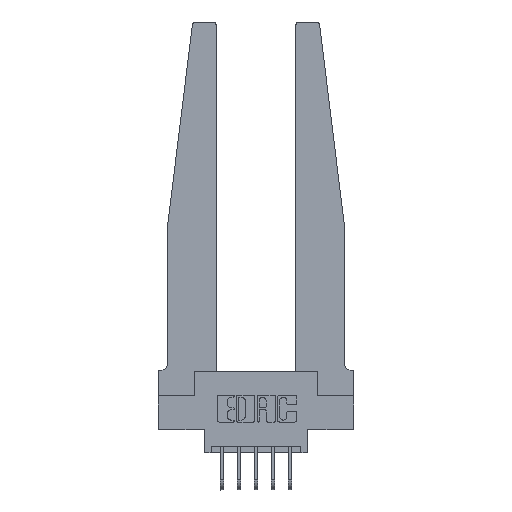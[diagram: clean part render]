
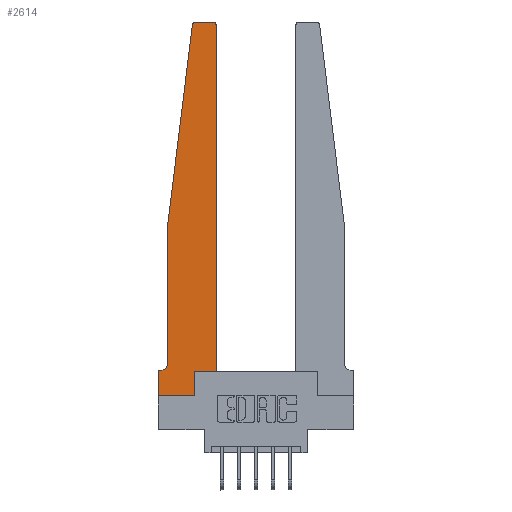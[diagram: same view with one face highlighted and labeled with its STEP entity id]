
A CAD part, top view. The second image highlights one B-rep face of the part: STEP entity #2614.
In plain terms, the highlighted planar face has unit normal (0, 0, 1).
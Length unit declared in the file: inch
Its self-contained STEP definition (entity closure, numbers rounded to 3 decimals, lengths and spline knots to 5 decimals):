
#94 = ORIENTED_EDGE ( 'NONE', *, *, #11833, .T. ) ;
#110 = DIRECTION ( 'NONE',  ( 0., 1., 0. ) ) ;
#205 = LINE ( 'NONE', #5189, #2556 ) ;
#256 = DIRECTION ( 'NONE',  ( 0., 1., 0. ) ) ;
#635 = EDGE_CURVE ( 'NONE', #6625, #7619, #13423, .T. ) ;
#731 = CARTESIAN_POINT ( 'NONE',  ( 0., 0.1875, 0.37 ) ) ;
#833 = CARTESIAN_POINT ( 'NONE',  ( 0.065, 1.25, 0.37 ) ) ;
#838 = VECTOR ( 'NONE', #7526, 39.37008 ) ;
#869 = ORIENTED_EDGE ( 'NONE', *, *, #635, .T. ) ;
#882 = EDGE_CURVE ( 'NONE', #1920, #13767, #6185, .T. ) ;
#1499 = VECTOR ( 'NONE', #4022, 39.37008 ) ;
#1547 = CARTESIAN_POINT ( 'NONE',  ( 0., 0., 0.37 ) ) ;
#1629 = DIRECTION ( 'NONE',  ( -1., 0., 0. ) ) ;
#1677 = CARTESIAN_POINT ( 'NONE',  ( 0.065, 1.25, 0.37 ) ) ;
#1782 = EDGE_CURVE ( 'NONE', #2402, #8370, #14694, .T. ) ;
#1840 = VERTEX_POINT ( 'NONE', #6152 ) ;
#1879 = ORIENTED_EDGE ( 'NONE', *, *, #11585, .T. ) ;
#1920 = VERTEX_POINT ( 'NONE', #11796 ) ;
#2402 = VERTEX_POINT ( 'NONE', #731 ) ;
#2556 = VECTOR ( 'NONE', #13270, 39.37008 ) ;
#2614 = ADVANCED_FACE ( 'NONE', ( #11369 ), #11522, .T. ) ;
#3141 = CARTESIAN_POINT ( 'NONE',  ( 0.27653, 2.75, 0.37 ) ) ;
#3259 = VECTOR ( 'NONE', #8153, 39.37008 ) ;
#3356 = VECTOR ( 'NONE', #110, 39.37008 ) ;
#3943 = VECTOR ( 'NONE', #256, 39.37008 ) ;
#3994 = ORIENTED_EDGE ( 'NONE', *, *, #15197, .T. ) ;
#4022 = DIRECTION ( 'NONE',  ( 1., 0., 0. ) ) ;
#4045 = DIRECTION ( 'NONE',  ( 0., -1., 0. ) ) ;
#4246 = EDGE_CURVE ( 'NONE', #13767, #1840, #205, .T. ) ;
#4521 = DIRECTION ( 'NONE',  ( 1., 0., 0. ) ) ;
#4933 = DIRECTION ( 'NONE',  ( -1., 0., 0. ) ) ;
#5189 = CARTESIAN_POINT ( 'NONE',  ( 0.425, 0.18, 0.37 ) ) ;
#5263 = CARTESIAN_POINT ( 'NONE',  ( 0.065, 1.25, 0.37 ) ) ;
#5547 = ORIENTED_EDGE ( 'NONE', *, *, #4246, .T. ) ;
#5619 = CARTESIAN_POINT ( 'NONE',  ( 0., 0.1875, 0.37 ) ) ;
#5696 = CARTESIAN_POINT ( 'NONE',  ( 0.27653, 2.72, 0.37 ) ) ;
#5888 = EDGE_CURVE ( 'NONE', #9339, #12869, #15027, .T. ) ;
#5959 = CARTESIAN_POINT ( 'NONE',  ( 0.2605, 0.18, 0.37 ) ) ;
#6021 = CARTESIAN_POINT ( 'NONE',  ( 0.065, 0.2375, 0.37 ) ) ;
#6118 = CARTESIAN_POINT ( 'NONE',  ( 0.395, 2.75, 0.37 ) ) ;
#6152 = CARTESIAN_POINT ( 'NONE',  ( 0.425, 0.18, 0.37 ) ) ;
#6185 = LINE ( 'NONE', #5959, #3356 ) ;
#6254 = CARTESIAN_POINT ( 'NONE',  ( 0.25, 2.75, 0.37 ) ) ;
#6352 = LINE ( 'NONE', #5263, #13363 ) ;
#6625 = VERTEX_POINT ( 'NONE', #12163 ) ;
#7405 = VECTOR ( 'NONE', #4045, 39.37008 ) ;
#7431 = LINE ( 'NONE', #6254, #14932 ) ;
#7526 = DIRECTION ( 'NONE',  ( -0.122, -0.992, 0. ) ) ;
#7563 = CARTESIAN_POINT ( 'NONE',  ( 0.015, 0.2375, 0.37 ) ) ;
#7589 = EDGE_CURVE ( 'NONE', #12134, #7979, #12583, .T. ) ;
#7619 = VERTEX_POINT ( 'NONE', #833 ) ;
#7979 = VERTEX_POINT ( 'NONE', #6118 ) ;
#8153 = DIRECTION ( 'NONE',  ( -1., 0., 0. ) ) ;
#8335 = AXIS2_PLACEMENT_3D ( 'NONE', #7563, #12303, #1629 ) ;
#8370 = VERTEX_POINT ( 'NONE', #8961 ) ;
#8431 = EDGE_CURVE ( 'NONE', #12006, #6625, #9137, .T. ) ;
#8456 = CARTESIAN_POINT ( 'NONE',  ( 0.425, 0.18, 0.37 ) ) ;
#8487 = ORIENTED_EDGE ( 'NONE', *, *, #882, .T. ) ;
#8545 = ORIENTED_EDGE ( 'NONE', *, *, #14710, .T. ) ;
#8605 = LINE ( 'NONE', #8456, #3943 ) ;
#8961 = CARTESIAN_POINT ( 'NONE',  ( 0., 0., 0.37 ) ) ;
#9137 = CIRCLE ( 'NONE', #11847, 0.03 ) ;
#9179 = DIRECTION ( 'NONE',  ( 1., 0., 0. ) ) ;
#9336 = ORIENTED_EDGE ( 'NONE', *, *, #8431, .T. ) ;
#9339 = VERTEX_POINT ( 'NONE', #6021 ) ;
#9862 = CARTESIAN_POINT ( 'NONE',  ( 0.395, 2.72, 0.37 ) ) ;
#9936 = LINE ( 'NONE', #14673, #1499 ) ;
#10217 = CARTESIAN_POINT ( 'NONE',  ( 0.425, 2.72, 0.37 ) ) ;
#10276 = DIRECTION ( 'NONE',  ( 0., 0., 1. ) ) ;
#10484 = LINE ( 'NONE', #11647, #3259 ) ;
#11335 = DIRECTION ( 'NONE',  ( 0., -1., 0. ) ) ;
#11369 = FACE_OUTER_BOUND ( 'NONE', #15198, .T. ) ;
#11522 = PLANE ( 'NONE',  #11664 ) ;
#11585 = EDGE_CURVE ( 'NONE', #7619, #9339, #6352, .T. ) ;
#11647 = CARTESIAN_POINT ( 'NONE',  ( 0.065, 0.1875, 0.37 ) ) ;
#11664 = AXIS2_PLACEMENT_3D ( 'NONE', #5619, #10276, #13697 ) ;
#11796 = CARTESIAN_POINT ( 'NONE',  ( 0.2605, 0., 0.37 ) ) ;
#11833 = EDGE_CURVE ( 'NONE', #1840, #12134, #8605, .T. ) ;
#11847 = AXIS2_PLACEMENT_3D ( 'NONE', #5696, #15165, #4521 ) ;
#12006 = VERTEX_POINT ( 'NONE', #3141 ) ;
#12134 = VERTEX_POINT ( 'NONE', #10217 ) ;
#12163 = CARTESIAN_POINT ( 'NONE',  ( 0.24675, 2.72367, 0.37 ) ) ;
#12303 = DIRECTION ( 'NONE',  ( 0., 0., -1. ) ) ;
#12583 = CIRCLE ( 'NONE', #13827, 0.03 ) ;
#12652 = ORIENTED_EDGE ( 'NONE', *, *, #1782, .T. ) ;
#12657 = CARTESIAN_POINT ( 'NONE',  ( 0.015, 0.1875, 0.37 ) ) ;
#12718 = ORIENTED_EDGE ( 'NONE', *, *, #5888, .T. ) ;
#12869 = VERTEX_POINT ( 'NONE', #12657 ) ;
#13270 = DIRECTION ( 'NONE',  ( 1., 0., 0. ) ) ;
#13363 = VECTOR ( 'NONE', #11335, 39.37008 ) ;
#13423 = LINE ( 'NONE', #1677, #838 ) ;
#13438 = CARTESIAN_POINT ( 'NONE',  ( 0.2605, 0.18, 0.37 ) ) ;
#13697 = DIRECTION ( 'NONE',  ( 1., 0., 0. ) ) ;
#13767 = VERTEX_POINT ( 'NONE', #13438 ) ;
#13827 = AXIS2_PLACEMENT_3D ( 'NONE', #9862, #14603, #9179 ) ;
#14258 = ORIENTED_EDGE ( 'NONE', *, *, #7589, .T. ) ;
#14603 = DIRECTION ( 'NONE',  ( 0., 0., 1. ) ) ;
#14642 = ORIENTED_EDGE ( 'NONE', *, *, #14919, .T. ) ;
#14673 = CARTESIAN_POINT ( 'NONE',  ( 0., 0., 0.37 ) ) ;
#14694 = LINE ( 'NONE', #1547, #7405 ) ;
#14710 = EDGE_CURVE ( 'NONE', #8370, #1920, #9936, .T. ) ;
#14919 = EDGE_CURVE ( 'NONE', #12869, #2402, #10484, .T. ) ;
#14932 = VECTOR ( 'NONE', #4933, 39.37008 ) ;
#15027 = CIRCLE ( 'NONE', #8335, 0.05 ) ;
#15165 = DIRECTION ( 'NONE',  ( 0., 0., 1. ) ) ;
#15197 = EDGE_CURVE ( 'NONE', #7979, #12006, #7431, .T. ) ;
#15198 = EDGE_LOOP ( 'NONE', ( #3994, #9336, #869, #1879, #12718, #14642, #12652, #8545, #8487, #5547, #94, #14258 ) ) ;
